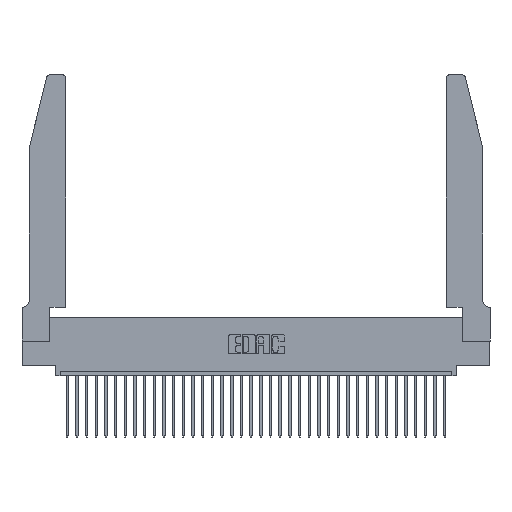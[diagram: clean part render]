
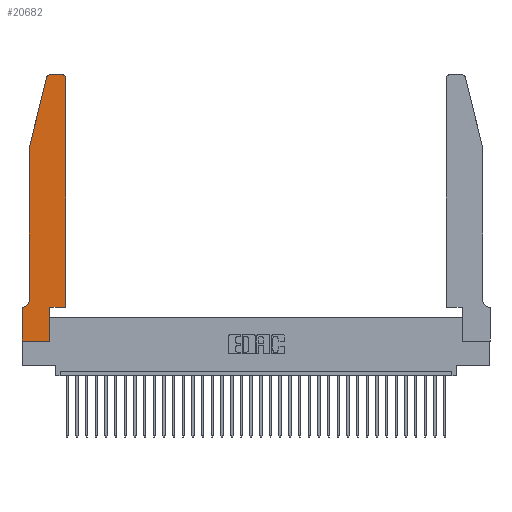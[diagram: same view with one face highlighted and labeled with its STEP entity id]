
A CAD part, top view. The second image highlights one B-rep face of the part: STEP entity #20682.
In plain terms, the highlighted planar face has unit normal (0, 0, 1).
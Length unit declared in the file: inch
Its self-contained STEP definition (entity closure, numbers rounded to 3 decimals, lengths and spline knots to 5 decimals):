
#84 = LINE ( 'NONE', #5919, #23962 ) ;
#86 = EDGE_CURVE ( 'NONE', #26562, #5685, #84, .T. ) ;
#301 = CIRCLE ( 'NONE', #3727, 0.03 ) ;
#709 = DIRECTION ( 'NONE',  ( 1., 0., 0. ) ) ;
#1239 = EDGE_CURVE ( 'NONE', #5685, #28152, #32404, .T. ) ;
#1554 = EDGE_CURVE ( 'NONE', #10012, #31642, #27669, .T. ) ;
#1609 = ORIENTED_EDGE ( 'NONE', *, *, #86, .T. ) ;
#1619 = CARTESIAN_POINT ( 'NONE',  ( 0.2865, 0.35, 0.37 ) ) ;
#1786 = DIRECTION ( 'NONE',  ( 0., -1., 0. ) ) ;
#1986 = VERTEX_POINT ( 'NONE', #25761 ) ;
#3003 = DIRECTION ( 'NONE',  ( 0., 1., 0. ) ) ;
#3262 = ORIENTED_EDGE ( 'NONE', *, *, #25976, .T. ) ;
#3313 = CARTESIAN_POINT ( 'NONE',  ( 0.284, 2.72, 0.37 ) ) ;
#3482 = CIRCLE ( 'NONE', #30608, 0.03 ) ;
#3727 = AXIS2_PLACEMENT_3D ( 'NONE', #3313, #24902, #16780 ) ;
#4028 = DIRECTION ( 'NONE',  ( 1., 0., 0. ) ) ;
#4061 = VECTOR ( 'NONE', #1786, 39.37008 ) ;
#4107 = EDGE_CURVE ( 'NONE', #28946, #22754, #16454, .T. ) ;
#4408 = CIRCLE ( 'NONE', #9136, 0.07 ) ;
#5020 = CARTESIAN_POINT ( 'NONE',  ( 0.0755, 2., 0.37 ) ) ;
#5685 = VERTEX_POINT ( 'NONE', #34149 ) ;
#5919 = CARTESIAN_POINT ( 'NONE',  ( 0.4505, 0.35, 0.37 ) ) ;
#6309 = ORIENTED_EDGE ( 'NONE', *, *, #16835, .T. ) ;
#6406 = DIRECTION ( 'NONE',  ( -0.239, -0.971, 0. ) ) ;
#6494 = DIRECTION ( 'NONE',  ( 1., 0., 0. ) ) ;
#8023 = AXIS2_PLACEMENT_3D ( 'NONE', #28352, #11553, #6494 ) ;
#8975 = CARTESIAN_POINT ( 'NONE',  ( 0.0755, 2., 0.37 ) ) ;
#9136 = AXIS2_PLACEMENT_3D ( 'NONE', #11957, #25507, #25152 ) ;
#9311 = PLANE ( 'NONE',  #8023 ) ;
#9626 = CARTESIAN_POINT ( 'NONE',  ( 0., 0., 0.37 ) ) ;
#9729 = VECTOR ( 'NONE', #18797, 39.37008 ) ;
#10012 = VERTEX_POINT ( 'NONE', #9626 ) ;
#10241 = VERTEX_POINT ( 'NONE', #29230 ) ;
#10358 = EDGE_CURVE ( 'NONE', #28152, #1986, #3482, .T. ) ;
#11433 = ORIENTED_EDGE ( 'NONE', *, *, #1239, .T. ) ;
#11553 = DIRECTION ( 'NONE',  ( 0., 0., 1. ) ) ;
#11677 = CARTESIAN_POINT ( 'NONE',  ( 0.0755, 2., 0.37 ) ) ;
#11693 = VERTEX_POINT ( 'NONE', #22635 ) ;
#11731 = ORIENTED_EDGE ( 'NONE', *, *, #32945, .T. ) ;
#11957 = CARTESIAN_POINT ( 'NONE',  ( 0.0055, 0.42, 0.37 ) ) ;
#12366 = LINE ( 'NONE', #5020, #22507 ) ;
#12830 = CARTESIAN_POINT ( 'NONE',  ( 0.4205, 2.72, 0.37 ) ) ;
#13064 = CARTESIAN_POINT ( 'NONE',  ( 0.4505, 2.72, 0.37 ) ) ;
#13117 = DIRECTION ( 'NONE',  ( 0., -1., 0. ) ) ;
#13485 = EDGE_CURVE ( 'NONE', #29491, #28946, #301, .T. ) ;
#13606 = ORIENTED_EDGE ( 'NONE', *, *, #32424, .T. ) ;
#13708 = LINE ( 'NONE', #30048, #16257 ) ;
#13763 = CARTESIAN_POINT ( 'NONE',  ( 0.284, 2.75, 0.37 ) ) ;
#14357 = VECTOR ( 'NONE', #6406, 39.37008 ) ;
#14874 = ORIENTED_EDGE ( 'NONE', *, *, #15786, .T. ) ;
#15060 = CARTESIAN_POINT ( 'NONE',  ( 0., 0.35, 0.37 ) ) ;
#15504 = CARTESIAN_POINT ( 'NONE',  ( 0.2865, 0., 0.37 ) ) ;
#15786 = EDGE_CURVE ( 'NONE', #1986, #29491, #28451, .T. ) ;
#16257 = VECTOR ( 'NONE', #33342, 39.37008 ) ;
#16454 = LINE ( 'NONE', #8975, #14357 ) ;
#16780 = DIRECTION ( 'NONE',  ( 1., 0., 0. ) ) ;
#16835 = EDGE_CURVE ( 'NONE', #18289, #10012, #35191, .T. ) ;
#17467 = ORIENTED_EDGE ( 'NONE', *, *, #18052, .T. ) ;
#17668 = ORIENTED_EDGE ( 'NONE', *, *, #4107, .T. ) ;
#18052 = EDGE_CURVE ( 'NONE', #11693, #10241, #4408, .T. ) ;
#18289 = VERTEX_POINT ( 'NONE', #15060 ) ;
#18674 = DIRECTION ( 'NONE',  ( 0., 0., 1. ) ) ;
#18797 = DIRECTION ( 'NONE',  ( 0., 1., 0. ) ) ;
#19070 = CARTESIAN_POINT ( 'NONE',  ( 0.4505, 0.35, 0.37 ) ) ;
#19099 = VECTOR ( 'NONE', #25989, 39.37008 ) ;
#19102 = DIRECTION ( 'NONE',  ( -1., 0., 0. ) ) ;
#20682 = ADVANCED_FACE ( 'NONE', ( #23880 ), #9311, .T. ) ;
#21832 = CARTESIAN_POINT ( 'NONE',  ( 0.25487, 2.72718, 0.37 ) ) ;
#22507 = VECTOR ( 'NONE', #13117, 39.37008 ) ;
#22635 = CARTESIAN_POINT ( 'NONE',  ( 0.0755, 0.42, 0.37 ) ) ;
#22684 = ORIENTED_EDGE ( 'NONE', *, *, #1554, .T. ) ;
#22754 = VERTEX_POINT ( 'NONE', #11677 ) ;
#23319 = ORIENTED_EDGE ( 'NONE', *, *, #13485, .T. ) ;
#23683 = CARTESIAN_POINT ( 'NONE',  ( 0., 0., 0.37 ) ) ;
#23770 = LINE ( 'NONE', #27181, #9729 ) ;
#23880 = FACE_OUTER_BOUND ( 'NONE', #25662, .T. ) ;
#23962 = VECTOR ( 'NONE', #709, 39.37008 ) ;
#24902 = DIRECTION ( 'NONE',  ( 0., 0., 1. ) ) ;
#25152 = DIRECTION ( 'NONE',  ( -1., 0., 0. ) ) ;
#25507 = DIRECTION ( 'NONE',  ( 0., 0., -1. ) ) ;
#25662 = EDGE_LOOP ( 'NONE', ( #14874, #23319, #17668, #13606, #17467, #3262, #6309, #22684, #11731, #1609, #11433, #28030 ) ) ;
#25761 = CARTESIAN_POINT ( 'NONE',  ( 0.4205, 2.75, 0.37 ) ) ;
#25976 = EDGE_CURVE ( 'NONE', #10241, #18289, #13708, .T. ) ;
#25989 = DIRECTION ( 'NONE',  ( 1., 0., 0. ) ) ;
#26562 = VERTEX_POINT ( 'NONE', #1619 ) ;
#27181 = CARTESIAN_POINT ( 'NONE',  ( 0.2865, 0.35, 0.37 ) ) ;
#27669 = LINE ( 'NONE', #30751, #19099 ) ;
#28030 = ORIENTED_EDGE ( 'NONE', *, *, #10358, .T. ) ;
#28152 = VERTEX_POINT ( 'NONE', #13064 ) ;
#28352 = CARTESIAN_POINT ( 'NONE',  ( 0., 0.35, 0.37 ) ) ;
#28451 = LINE ( 'NONE', #31728, #30146 ) ;
#28946 = VERTEX_POINT ( 'NONE', #21832 ) ;
#29230 = CARTESIAN_POINT ( 'NONE',  ( 0.0055, 0.35, 0.37 ) ) ;
#29491 = VERTEX_POINT ( 'NONE', #13763 ) ;
#30048 = CARTESIAN_POINT ( 'NONE',  ( 0.0755, 0.35, 0.37 ) ) ;
#30146 = VECTOR ( 'NONE', #19102, 39.37008 ) ;
#30608 = AXIS2_PLACEMENT_3D ( 'NONE', #12830, #18674, #4028 ) ;
#30693 = VECTOR ( 'NONE', #3003, 39.37008 ) ;
#30751 = CARTESIAN_POINT ( 'NONE',  ( 0., 0., 0.37 ) ) ;
#31642 = VERTEX_POINT ( 'NONE', #15504 ) ;
#31728 = CARTESIAN_POINT ( 'NONE',  ( 0.2605, 2.75, 0.37 ) ) ;
#32404 = LINE ( 'NONE', #19070, #30693 ) ;
#32424 = EDGE_CURVE ( 'NONE', #22754, #11693, #12366, .T. ) ;
#32945 = EDGE_CURVE ( 'NONE', #31642, #26562, #23770, .T. ) ;
#33342 = DIRECTION ( 'NONE',  ( -1., 0., 0. ) ) ;
#34149 = CARTESIAN_POINT ( 'NONE',  ( 0.4505, 0.35, 0.37 ) ) ;
#35191 = LINE ( 'NONE', #23683, #4061 ) ;
